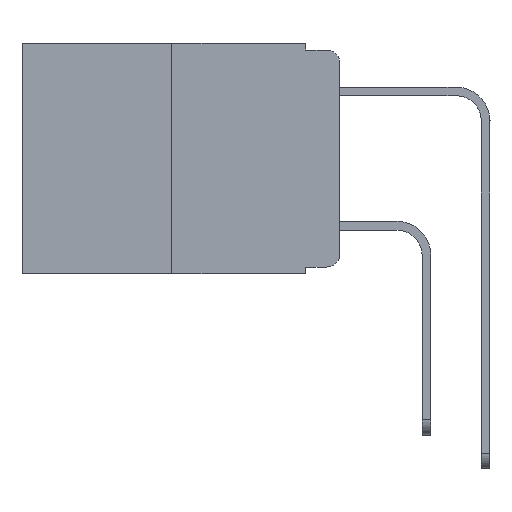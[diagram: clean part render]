
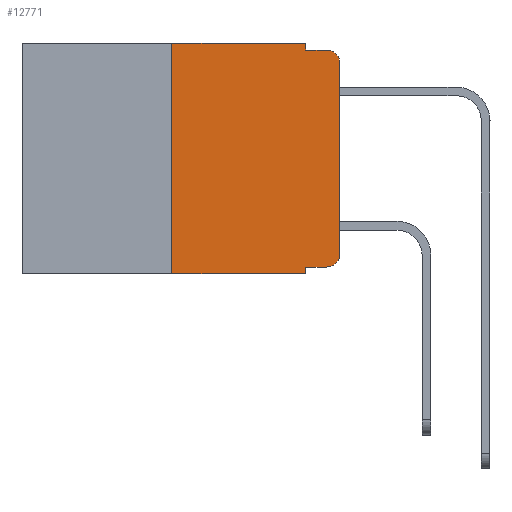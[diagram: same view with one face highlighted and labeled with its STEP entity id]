
A CAD part, left-side view. The second image highlights one B-rep face of the part: STEP entity #12771.
In plain terms, the highlighted planar face has unit normal (-1, 0, 0).
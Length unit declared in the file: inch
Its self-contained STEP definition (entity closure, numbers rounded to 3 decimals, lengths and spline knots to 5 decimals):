
#26 = CIRCLE ( 'NONE', #1654, 0.02 ) ;
#171 = EDGE_CURVE ( 'NONE', #8035, #4702, #10171, .T. ) ;
#300 = DIRECTION ( 'NONE',  ( -1., 0., 0. ) ) ;
#551 = CARTESIAN_POINT ( 'NONE',  ( 0., 0.051, -0.333 ) ) ;
#822 = ORIENTED_EDGE ( 'NONE', *, *, #6615, .T. ) ;
#828 = EDGE_LOOP ( 'NONE', ( #14385, #3653, #3453, #9239, #13767, #8101, #5414, #7019, #3918, #822 ) ) ;
#899 = DIRECTION ( 'NONE',  ( 0., 0., -1. ) ) ;
#1058 = CARTESIAN_POINT ( 'NONE',  ( 0., 0.051, -0.343 ) ) ;
#1347 = CARTESIAN_POINT ( 'NONE',  ( 0., 0.051, -0.01 ) ) ;
#1654 = AXIS2_PLACEMENT_3D ( 'NONE', #7203, #300, #8320 ) ;
#1687 = EDGE_CURVE ( 'NONE', #2281, #13799, #2227, .T. ) ;
#1726 = CARTESIAN_POINT ( 'NONE',  ( 0., 0.051, 0. ) ) ;
#1731 = VECTOR ( 'NONE', #13790, 39.37008 ) ;
#2198 = VECTOR ( 'NONE', #8203, 39.37008 ) ;
#2227 = LINE ( 'NONE', #8071, #10485 ) ;
#2242 = EDGE_CURVE ( 'NONE', #8045, #13585, #11150, .T. ) ;
#2281 = VERTEX_POINT ( 'NONE', #2613 ) ;
#2443 = VECTOR ( 'NONE', #8148, 39.37008 ) ;
#2508 = CARTESIAN_POINT ( 'NONE',  ( 0., 0.473, -0.343 ) ) ;
#2533 = LINE ( 'NONE', #13954, #5219 ) ;
#2596 = LINE ( 'NONE', #2508, #2443 ) ;
#2606 = EDGE_CURVE ( 'NONE', #8035, #10316, #6729, .T. ) ;
#2613 = CARTESIAN_POINT ( 'NONE',  ( 0., 0., -0.313 ) ) ;
#2902 = EDGE_CURVE ( 'NONE', #13799, #13585, #26, .T. ) ;
#3135 = CARTESIAN_POINT ( 'NONE',  ( 0., 0.25, 0. ) ) ;
#3453 = ORIENTED_EDGE ( 'NONE', *, *, #2242, .F. ) ;
#3653 = ORIENTED_EDGE ( 'NONE', *, *, #2902, .T. ) ;
#3770 = VECTOR ( 'NONE', #7791, 39.37008 ) ;
#3918 = ORIENTED_EDGE ( 'NONE', *, *, #171, .T. ) ;
#4163 = CARTESIAN_POINT ( 'NONE',  ( 0., 0.051, -0.01 ) ) ;
#4251 = VECTOR ( 'NONE', #13000, 39.37008 ) ;
#4405 = PLANE ( 'NONE',  #11295 ) ;
#4552 = EDGE_CURVE ( 'NONE', #9009, #10316, #2596, .T. ) ;
#4702 = VERTEX_POINT ( 'NONE', #7310 ) ;
#4833 = LINE ( 'NONE', #7153, #1731 ) ;
#5219 = VECTOR ( 'NONE', #11717, 39.37008 ) ;
#5414 = ORIENTED_EDGE ( 'NONE', *, *, #4552, .T. ) ;
#6486 = VERTEX_POINT ( 'NONE', #1726 ) ;
#6525 = DIRECTION ( 'NONE',  ( -1., 0., 0. ) ) ;
#6615 = EDGE_CURVE ( 'NONE', #4702, #2281, #12735, .T. ) ;
#6729 = LINE ( 'NONE', #12206, #3770 ) ;
#7019 = ORIENTED_EDGE ( 'NONE', *, *, #2606, .F. ) ;
#7153 = CARTESIAN_POINT ( 'NONE',  ( 0., 0.473, 0. ) ) ;
#7203 = CARTESIAN_POINT ( 'NONE',  ( 0., 0.02, -0.03 ) ) ;
#7310 = CARTESIAN_POINT ( 'NONE',  ( 0., 0.02, -0.333 ) ) ;
#7714 = AXIS2_PLACEMENT_3D ( 'NONE', #13181, #6525, #14284 ) ;
#7763 = DIRECTION ( 'NONE',  ( 1., 0., 0. ) ) ;
#7791 = DIRECTION ( 'NONE',  ( 0., 0., -1. ) ) ;
#8035 = VERTEX_POINT ( 'NONE', #551 ) ;
#8045 = VERTEX_POINT ( 'NONE', #4163 ) ;
#8071 = CARTESIAN_POINT ( 'NONE',  ( 0., 0., 0. ) ) ;
#8101 = ORIENTED_EDGE ( 'NONE', *, *, #11333, .F. ) ;
#8148 = DIRECTION ( 'NONE',  ( 0., -1., 0. ) ) ;
#8203 = DIRECTION ( 'NONE',  ( 0., -1., 0. ) ) ;
#8278 = CARTESIAN_POINT ( 'NONE',  ( 0., 0., -0.03 ) ) ;
#8320 = DIRECTION ( 'NONE',  ( 0., 0., -1. ) ) ;
#9009 = VERTEX_POINT ( 'NONE', #11376 ) ;
#9187 = DIRECTION ( 'NONE',  ( 0., 0., 1. ) ) ;
#9239 = ORIENTED_EDGE ( 'NONE', *, *, #13120, .F. ) ;
#9846 = DIRECTION ( 'NONE',  ( 0., 0., 1. ) ) ;
#9848 = EDGE_CURVE ( 'NONE', #11660, #6486, #4833, .T. ) ;
#9913 = FACE_OUTER_BOUND ( 'NONE', #828, .T. ) ;
#10171 = LINE ( 'NONE', #11990, #4251 ) ;
#10316 = VERTEX_POINT ( 'NONE', #1058 ) ;
#10402 = CARTESIAN_POINT ( 'NONE',  ( 0., 0.25, 0. ) ) ;
#10485 = VECTOR ( 'NONE', #9187, 39.37008 ) ;
#11047 = CARTESIAN_POINT ( 'NONE',  ( 0., 0.473, 0. ) ) ;
#11150 = LINE ( 'NONE', #1347, #2198 ) ;
#11295 = AXIS2_PLACEMENT_3D ( 'NONE', #11047, #7763, #899 ) ;
#11333 = EDGE_CURVE ( 'NONE', #9009, #11660, #13425, .T. ) ;
#11376 = CARTESIAN_POINT ( 'NONE',  ( 0., 0.25, -0.343 ) ) ;
#11660 = VERTEX_POINT ( 'NONE', #10402 ) ;
#11717 = DIRECTION ( 'NONE',  ( 0., 0., -1. ) ) ;
#11990 = CARTESIAN_POINT ( 'NONE',  ( 0., 0.051, -0.333 ) ) ;
#12206 = CARTESIAN_POINT ( 'NONE',  ( 0., 0.051, 0. ) ) ;
#12735 = CIRCLE ( 'NONE', #7714, 0.02 ) ;
#12771 = ADVANCED_FACE ( 'NONE', ( #9913 ), #4405, .F. ) ;
#13000 = DIRECTION ( 'NONE',  ( 0., -1., 0. ) ) ;
#13070 = VECTOR ( 'NONE', #9846, 39.37008 ) ;
#13120 = EDGE_CURVE ( 'NONE', #6486, #8045, #2533, .T. ) ;
#13181 = CARTESIAN_POINT ( 'NONE',  ( 0., 0.02, -0.313 ) ) ;
#13425 = LINE ( 'NONE', #3135, #13070 ) ;
#13585 = VERTEX_POINT ( 'NONE', #14557 ) ;
#13767 = ORIENTED_EDGE ( 'NONE', *, *, #9848, .F. ) ;
#13790 = DIRECTION ( 'NONE',  ( 0., -1., 0. ) ) ;
#13799 = VERTEX_POINT ( 'NONE', #8278 ) ;
#13954 = CARTESIAN_POINT ( 'NONE',  ( 0., 0.051, 0. ) ) ;
#14284 = DIRECTION ( 'NONE',  ( 0., 0., -1. ) ) ;
#14385 = ORIENTED_EDGE ( 'NONE', *, *, #1687, .T. ) ;
#14557 = CARTESIAN_POINT ( 'NONE',  ( 0., 0.02, -0.01 ) ) ;
